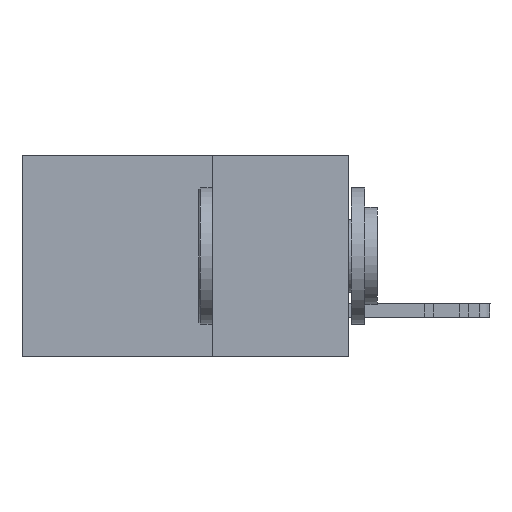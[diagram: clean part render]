
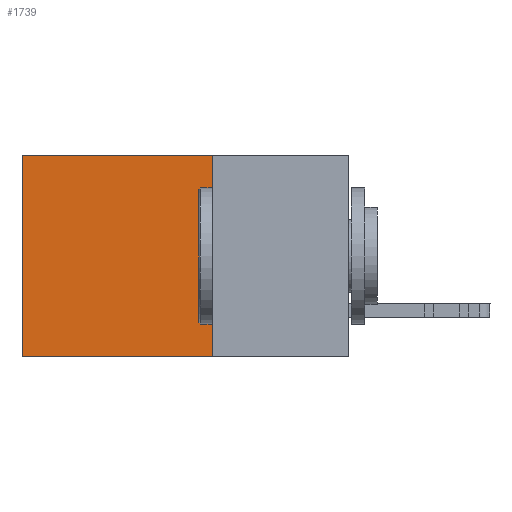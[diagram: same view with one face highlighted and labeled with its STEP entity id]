
A CAD part, left-side view. The second image highlights one B-rep face of the part: STEP entity #1739.
In plain terms, the highlighted planar face has unit normal (-1, 0, 0).
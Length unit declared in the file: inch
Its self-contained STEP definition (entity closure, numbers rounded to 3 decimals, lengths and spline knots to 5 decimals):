
#1413 = LINE ( 'NONE', #8786, #16308 ) ;
#1739 = ADVANCED_FACE ( 'NONE', ( #21702 ), #23822, .F. ) ;
#3438 = CARTESIAN_POINT ( 'NONE',  ( 0.2615, 0.25, 0. ) ) ;
#4471 = AXIS2_PLACEMENT_3D ( 'NONE', #5134, #5232, #7364 ) ;
#4547 = CARTESIAN_POINT ( 'NONE',  ( 0.2615, 0.25, 0. ) ) ;
#5134 = CARTESIAN_POINT ( 'NONE',  ( 0.2615, 0.25, -0.37 ) ) ;
#5232 = DIRECTION ( 'NONE',  ( 1., 0., 0. ) ) ;
#6552 = VERTEX_POINT ( 'NONE', #4547 ) ;
#7073 = LINE ( 'NONE', #3438, #14263 ) ;
#7364 = DIRECTION ( 'NONE',  ( 0., 0., -1. ) ) ;
#8786 = CARTESIAN_POINT ( 'NONE',  ( 0.2615, 0.25, -0.37 ) ) ;
#9249 = VECTOR ( 'NONE', #15175, 39.37008 ) ;
#9378 = VERTEX_POINT ( 'NONE', #12817 ) ;
#9568 = CARTESIAN_POINT ( 'NONE',  ( 0.2615, 0.6, -0.37 ) ) ;
#9881 = LINE ( 'NONE', #19092, #21381 ) ;
#10242 = ORIENTED_EDGE ( 'NONE', *, *, #17949, .F. ) ;
#11658 = ORIENTED_EDGE ( 'NONE', *, *, #22879, .T. ) ;
#11769 = ORIENTED_EDGE ( 'NONE', *, *, #20503, .F. ) ;
#12817 = CARTESIAN_POINT ( 'NONE',  ( 0.2615, 0.6, 0. ) ) ;
#14263 = VECTOR ( 'NONE', #14556, 39.37008 ) ;
#14556 = DIRECTION ( 'NONE',  ( 0., 1., 0. ) ) ;
#15175 = DIRECTION ( 'NONE',  ( 0., 1., 0. ) ) ;
#15664 = VERTEX_POINT ( 'NONE', #9568 ) ;
#16308 = VECTOR ( 'NONE', #22905, 39.37008 ) ;
#17949 = EDGE_CURVE ( 'NONE', #21476, #15664, #18929, .T. ) ;
#18929 = LINE ( 'NONE', #19061, #9249 ) ;
#19061 = CARTESIAN_POINT ( 'NONE',  ( 0.2615, 0.25, -0.37 ) ) ;
#19092 = CARTESIAN_POINT ( 'NONE',  ( 0.2615, 0.6, -0.37 ) ) ;
#19793 = EDGE_LOOP ( 'NONE', ( #11658, #10242, #11769, #23661 ) ) ;
#20503 = EDGE_CURVE ( 'NONE', #6552, #21476, #1413, .T. ) ;
#21381 = VECTOR ( 'NONE', #22941, 39.37008 ) ;
#21476 = VERTEX_POINT ( 'NONE', #22216 ) ;
#21702 = FACE_OUTER_BOUND ( 'NONE', #19793, .T. ) ;
#22216 = CARTESIAN_POINT ( 'NONE',  ( 0.2615, 0.25, -0.37 ) ) ;
#22879 = EDGE_CURVE ( 'NONE', #9378, #15664, #9881, .T. ) ;
#22905 = DIRECTION ( 'NONE',  ( 0., 0., -1. ) ) ;
#22941 = DIRECTION ( 'NONE',  ( 0., 0., -1. ) ) ;
#23661 = ORIENTED_EDGE ( 'NONE', *, *, #23838, .T. ) ;
#23822 = PLANE ( 'NONE',  #4471 ) ;
#23838 = EDGE_CURVE ( 'NONE', #6552, #9378, #7073, .T. ) ;
